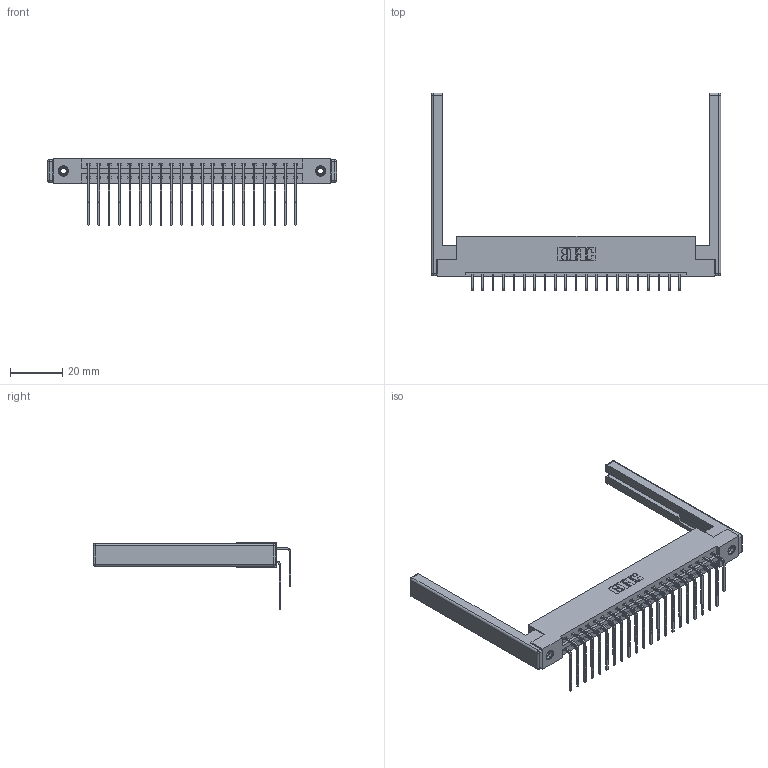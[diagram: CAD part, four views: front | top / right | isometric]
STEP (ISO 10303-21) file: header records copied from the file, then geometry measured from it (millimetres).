
FILE_DESCRIPTION (( 'STEP AP203' ), '1' );
FILE_NAME ('387-042-559-268.STEP', '2019-10-18T04:52:41', ( '' ), ( '' ), 'SwSTEP 2.0', 'SolidWorks 2016', '' );
FILE_SCHEMA (( 'CONFIG_CONTROL_DESIGN' ));
Length unit declared in the file: inch
Products named in the file (6): 307-220-068; 337 Part_Flush Mounting Lugs - 0.156 Dia-TI; 387-042-559-268; 345-292-001_558 559 Tail - 1; 345-250-001_345-250-001-102; 345-292-001_559 Tail - 2
Assembly tree (47 placements, depth 2):
  387-042-559-268
    337 Part_Flush Mounting Lugs - 0.156 Dia-TI
    345-292-001_558 559 Tail - 1  x21
    345-292-001_559 Tail - 2  x21
    345-250-001_345-250-001-102  x2
    307-220-068  x2
Bounding box: 110.64 x 75.63 x 25.53 mm (x, y, z)
Volume: 16007.9 mm3; surface area: 18186.9 mm2
Topology: 47 solids, 47 shells, 2620 faces, 7715 edges, 5066 vertices
Faces by surface type: plane 1838, cylinder 758, cone 12, sphere 8, torus 4
Entity records: 23542 total; most frequent: CARTESIAN_POINT 3994, ORIENTED_EDGE 3868, DIRECTION 3488, EDGE_CURVE 1934, LINE 1716, VECTOR 1716, VERTEX_POINT 1278, AXIS2_PLACEMENT_3D 886
